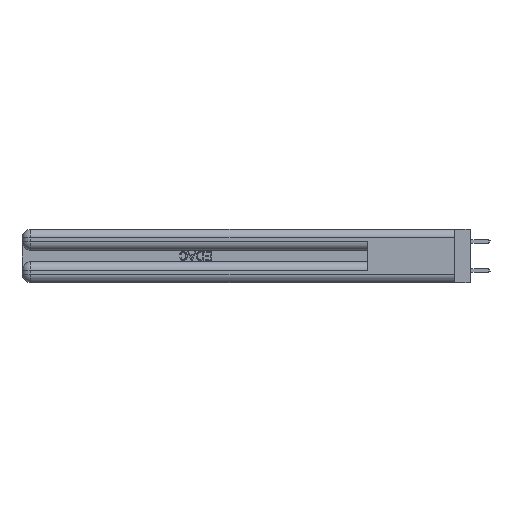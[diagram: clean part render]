
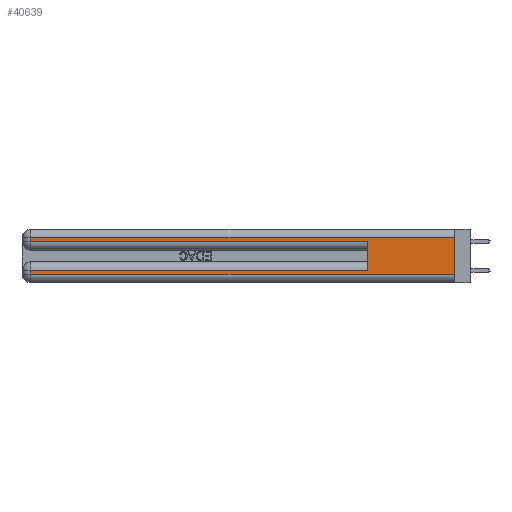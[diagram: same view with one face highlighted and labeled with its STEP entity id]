
A CAD part, left-side view. The second image highlights one B-rep face of the part: STEP entity #40639.
In plain terms, the highlighted planar face has unit normal (-1, 0, 0).
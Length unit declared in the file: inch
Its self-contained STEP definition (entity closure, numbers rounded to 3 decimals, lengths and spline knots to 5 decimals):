
#728 = DIRECTION ( 'NONE',  ( 0., 1., 0. ) ) ;
#1121 = ORIENTED_EDGE ( 'NONE', *, *, #21179, .F. ) ;
#2579 = VECTOR ( 'NONE', #8059, 39.37008 ) ;
#2620 = VECTOR ( 'NONE', #28152, 39.37008 ) ;
#2631 = AXIS2_PLACEMENT_3D ( 'NONE', #45014, #22321, #48769 ) ;
#3422 = VERTEX_POINT ( 'NONE', #48165 ) ;
#3623 = EDGE_CURVE ( 'NONE', #24871, #48390, #33894, .T. ) ;
#3628 = CARTESIAN_POINT ( 'NONE',  ( 0., 0.6, 0.285 ) ) ;
#3694 = CARTESIAN_POINT ( 'NONE',  ( 0., 2.94, 0.37 ) ) ;
#4156 = VECTOR ( 'NONE', #19398, 39.37008 ) ;
#4587 = VECTOR ( 'NONE', #45529, 39.37008 ) ;
#4677 = CARTESIAN_POINT ( 'NONE',  ( 0., 2.94, 0.085 ) ) ;
#5014 = LINE ( 'NONE', #34776, #2579 ) ;
#6567 = ORIENTED_EDGE ( 'NONE', *, *, #8527, .T. ) ;
#7799 = EDGE_CURVE ( 'NONE', #18607, #13531, #31778, .T. ) ;
#8059 = DIRECTION ( 'NONE',  ( 0., -1., 0. ) ) ;
#8067 = EDGE_CURVE ( 'NONE', #13531, #3422, #41239, .T. ) ;
#8337 = CARTESIAN_POINT ( 'NONE',  ( 0., 0., 0.085 ) ) ;
#8527 = EDGE_CURVE ( 'NONE', #3422, #14334, #13235, .T. ) ;
#9922 = CARTESIAN_POINT ( 'NONE',  ( 0., 2.94, 0.31 ) ) ;
#10419 = LINE ( 'NONE', #45488, #39664 ) ;
#11482 = VECTOR ( 'NONE', #15593, 39.37008 ) ;
#11874 = EDGE_CURVE ( 'NONE', #18607, #32730, #10419, .T. ) ;
#12914 = ORIENTED_EDGE ( 'NONE', *, *, #7799, .T. ) ;
#13235 = LINE ( 'NONE', #45878, #4156 ) ;
#13525 = VECTOR ( 'NONE', #728, 39.37008 ) ;
#13531 = VERTEX_POINT ( 'NONE', #9922 ) ;
#14334 = VERTEX_POINT ( 'NONE', #3628 ) ;
#15593 = DIRECTION ( 'NONE',  ( 0., 1., 0. ) ) ;
#15647 = CARTESIAN_POINT ( 'NONE',  ( 0., 0., 0.31 ) ) ;
#16158 = CARTESIAN_POINT ( 'NONE',  ( 0., 0., 0.06 ) ) ;
#17271 = ORIENTED_EDGE ( 'NONE', *, *, #3623, .T. ) ;
#18607 = VERTEX_POINT ( 'NONE', #15647 ) ;
#19398 = DIRECTION ( 'NONE',  ( 0., -1., 0. ) ) ;
#19470 = EDGE_LOOP ( 'NONE', ( #22368, #12914, #40603, #6567, #1121, #45805, #17271, #31497 ) ) ;
#20512 = CARTESIAN_POINT ( 'NONE',  ( 0., 0.6, 0.145 ) ) ;
#20743 = CARTESIAN_POINT ( 'NONE',  ( 0., 2.94, 0.06 ) ) ;
#21179 = EDGE_CURVE ( 'NONE', #47057, #14334, #33141, .T. ) ;
#22321 = DIRECTION ( 'NONE',  ( 1., 0., 0. ) ) ;
#22368 = ORIENTED_EDGE ( 'NONE', *, *, #11874, .F. ) ;
#24807 = EDGE_CURVE ( 'NONE', #48390, #32730, #5014, .T. ) ;
#24871 = VERTEX_POINT ( 'NONE', #4677 ) ;
#26941 = CARTESIAN_POINT ( 'NONE',  ( 0., 0., 0.31 ) ) ;
#28152 = DIRECTION ( 'NONE',  ( 0., 0., 1. ) ) ;
#31163 = VECTOR ( 'NONE', #43478, 39.37008 ) ;
#31497 = ORIENTED_EDGE ( 'NONE', *, *, #24807, .T. ) ;
#31778 = LINE ( 'NONE', #26941, #11482 ) ;
#32730 = VERTEX_POINT ( 'NONE', #16158 ) ;
#32815 = FACE_OUTER_BOUND ( 'NONE', #19470, .T. ) ;
#33141 = LINE ( 'NONE', #20512, #2620 ) ;
#33894 = LINE ( 'NONE', #3694, #4587 ) ;
#34776 = CARTESIAN_POINT ( 'NONE',  ( 0., 0., 0.06 ) ) ;
#37147 = EDGE_CURVE ( 'NONE', #47057, #24871, #43862, .T. ) ;
#37418 = PLANE ( 'NONE',  #2631 ) ;
#39664 = VECTOR ( 'NONE', #41892, 39.37008 ) ;
#39670 = CARTESIAN_POINT ( 'NONE',  ( 0., 2.94, 0.37 ) ) ;
#40603 = ORIENTED_EDGE ( 'NONE', *, *, #8067, .T. ) ;
#40639 = ADVANCED_FACE ( 'NONE', ( #32815 ), #37418, .F. ) ;
#41239 = LINE ( 'NONE', #39670, #31163 ) ;
#41892 = DIRECTION ( 'NONE',  ( 0., 0., -1. ) ) ;
#42899 = CARTESIAN_POINT ( 'NONE',  ( 0., 0.6, 0.085 ) ) ;
#43478 = DIRECTION ( 'NONE',  ( 0., 0., -1. ) ) ;
#43862 = LINE ( 'NONE', #8337, #13525 ) ;
#45014 = CARTESIAN_POINT ( 'NONE',  ( 0., 0., 0.37 ) ) ;
#45488 = CARTESIAN_POINT ( 'NONE',  ( 0., 0., 0.37 ) ) ;
#45529 = DIRECTION ( 'NONE',  ( 0., 0., -1. ) ) ;
#45805 = ORIENTED_EDGE ( 'NONE', *, *, #37147, .T. ) ;
#45878 = CARTESIAN_POINT ( 'NONE',  ( 0., 0., 0.285 ) ) ;
#47057 = VERTEX_POINT ( 'NONE', #42899 ) ;
#48165 = CARTESIAN_POINT ( 'NONE',  ( 0., 2.94, 0.285 ) ) ;
#48390 = VERTEX_POINT ( 'NONE', #20743 ) ;
#48769 = DIRECTION ( 'NONE',  ( 0., 0., -1. ) ) ;
